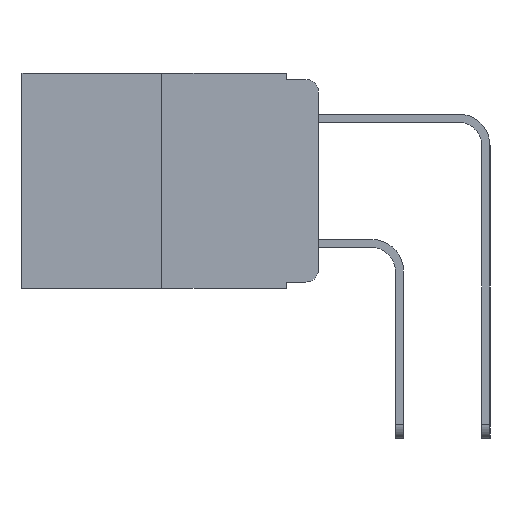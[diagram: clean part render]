
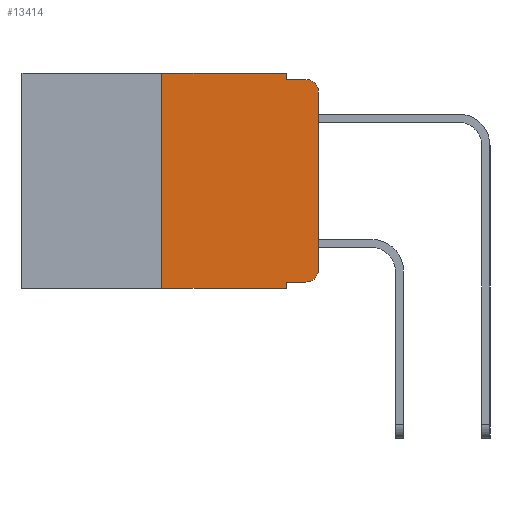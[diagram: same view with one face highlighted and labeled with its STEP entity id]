
A CAD part, left-side view. The second image highlights one B-rep face of the part: STEP entity #13414.
In plain terms, the highlighted planar face has unit normal (-1, 0, 0).
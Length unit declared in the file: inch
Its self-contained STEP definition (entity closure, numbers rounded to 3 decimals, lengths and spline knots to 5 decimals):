
#499 = LINE ( 'NONE', #9097, #16905 ) ;
#1325 = CARTESIAN_POINT ( 'NONE',  ( 0., 0., 0. ) ) ;
#1436 = PLANE ( 'NONE',  #6211 ) ;
#1549 = FACE_OUTER_BOUND ( 'NONE', #18176, .T. ) ;
#1709 = DIRECTION ( 'NONE',  ( 0., 0., -1. ) ) ;
#2256 = VERTEX_POINT ( 'NONE', #17069 ) ;
#2595 = DIRECTION ( 'NONE',  ( 0., 0., -1. ) ) ;
#2981 = CARTESIAN_POINT ( 'NONE',  ( 0., 0.051, -0.01 ) ) ;
#3268 = CARTESIAN_POINT ( 'NONE',  ( 0., 0.02, -0.313 ) ) ;
#3445 = EDGE_CURVE ( 'NONE', #6147, #6642, #19746, .T. ) ;
#4280 = LINE ( 'NONE', #12905, #16364 ) ;
#4606 = VERTEX_POINT ( 'NONE', #10904 ) ;
#4741 = DIRECTION ( 'NONE',  ( 1., 0., 0. ) ) ;
#4770 = ORIENTED_EDGE ( 'NONE', *, *, #20337, .T. ) ;
#4791 = ORIENTED_EDGE ( 'NONE', *, *, #17960, .T. ) ;
#4918 = DIRECTION ( 'NONE',  ( 0., 0., -1. ) ) ;
#5197 = AXIS2_PLACEMENT_3D ( 'NONE', #3268, #14366, #4918 ) ;
#5514 = EDGE_CURVE ( 'NONE', #6147, #6478, #12520, .T. ) ;
#5603 = EDGE_CURVE ( 'NONE', #6843, #2256, #10589, .T. ) ;
#5660 = CARTESIAN_POINT ( 'NONE',  ( 0., 0., -0.03 ) ) ;
#5936 = VERTEX_POINT ( 'NONE', #14163 ) ;
#6147 = VERTEX_POINT ( 'NONE', #11583 ) ;
#6211 = AXIS2_PLACEMENT_3D ( 'NONE', #17232, #4741, #15773 ) ;
#6478 = VERTEX_POINT ( 'NONE', #17294 ) ;
#6642 = VERTEX_POINT ( 'NONE', #16165 ) ;
#6843 = VERTEX_POINT ( 'NONE', #5660 ) ;
#7044 = DIRECTION ( 'NONE',  ( -1., 0., 0. ) ) ;
#7381 = VECTOR ( 'NONE', #11989, 39.37008 ) ;
#7773 = CARTESIAN_POINT ( 'NONE',  ( 0., 0., -0.313 ) ) ;
#8070 = ORIENTED_EDGE ( 'NONE', *, *, #19618, .T. ) ;
#8300 = ORIENTED_EDGE ( 'NONE', *, *, #10717, .F. ) ;
#9097 = CARTESIAN_POINT ( 'NONE',  ( 0., 0.051, -0.333 ) ) ;
#9111 = CARTESIAN_POINT ( 'NONE',  ( 0., 0.051, 0. ) ) ;
#9526 = VERTEX_POINT ( 'NONE', #2981 ) ;
#10340 = CARTESIAN_POINT ( 'NONE',  ( 0., 0.473, -0.343 ) ) ;
#10366 = DIRECTION ( 'NONE',  ( 0., -1., 0. ) ) ;
#10451 = CARTESIAN_POINT ( 'NONE',  ( 0., 0.051, -0.01 ) ) ;
#10589 = CIRCLE ( 'NONE', #18499, 0.02 ) ;
#10717 = EDGE_CURVE ( 'NONE', #4606, #9526, #20004, .T. ) ;
#10824 = VERTEX_POINT ( 'NONE', #7773 ) ;
#10904 = CARTESIAN_POINT ( 'NONE',  ( 0., 0.051, 0. ) ) ;
#11104 = VECTOR ( 'NONE', #10366, 39.37008 ) ;
#11280 = ORIENTED_EDGE ( 'NONE', *, *, #15408, .F. ) ;
#11535 = CARTESIAN_POINT ( 'NONE',  ( 0., 0.25, 0. ) ) ;
#11583 = CARTESIAN_POINT ( 'NONE',  ( 0., 0.25, -0.343 ) ) ;
#11989 = DIRECTION ( 'NONE',  ( 0., -1., 0. ) ) ;
#12031 = VECTOR ( 'NONE', #13077, 39.37008 ) ;
#12056 = LINE ( 'NONE', #10451, #7381 ) ;
#12410 = EDGE_CURVE ( 'NONE', #9526, #2256, #12056, .T. ) ;
#12520 = LINE ( 'NONE', #11535, #12031 ) ;
#12905 = CARTESIAN_POINT ( 'NONE',  ( 0., 0.051, 0. ) ) ;
#13077 = DIRECTION ( 'NONE',  ( 0., 0., 1. ) ) ;
#13414 = ADVANCED_FACE ( 'NONE', ( #1549 ), #1436, .F. ) ;
#13696 = ORIENTED_EDGE ( 'NONE', *, *, #5603, .T. ) ;
#13946 = ORIENTED_EDGE ( 'NONE', *, *, #17488, .F. ) ;
#14104 = DIRECTION ( 'NONE',  ( 0., 0., 1. ) ) ;
#14163 = CARTESIAN_POINT ( 'NONE',  ( 0., 0.02, -0.333 ) ) ;
#14366 = DIRECTION ( 'NONE',  ( -1., 0., 0. ) ) ;
#14423 = ORIENTED_EDGE ( 'NONE', *, *, #5514, .F. ) ;
#15408 = EDGE_CURVE ( 'NONE', #17806, #6642, #4280, .T. ) ;
#15773 = DIRECTION ( 'NONE',  ( 0., 0., -1. ) ) ;
#16165 = CARTESIAN_POINT ( 'NONE',  ( 0., 0.051, -0.343 ) ) ;
#16364 = VECTOR ( 'NONE', #1709, 39.37008 ) ;
#16402 = CARTESIAN_POINT ( 'NONE',  ( 0., 0.02, -0.03 ) ) ;
#16905 = VECTOR ( 'NONE', #18346, 39.37008 ) ;
#17069 = CARTESIAN_POINT ( 'NONE',  ( 0., 0.02, -0.01 ) ) ;
#17232 = CARTESIAN_POINT ( 'NONE',  ( 0., 0.473, 0. ) ) ;
#17294 = CARTESIAN_POINT ( 'NONE',  ( 0., 0.25, 0. ) ) ;
#17462 = CIRCLE ( 'NONE', #5197, 0.02 ) ;
#17488 = EDGE_CURVE ( 'NONE', #6478, #4606, #18435, .T. ) ;
#17799 = CARTESIAN_POINT ( 'NONE',  ( 0., 0.473, 0. ) ) ;
#17806 = VERTEX_POINT ( 'NONE', #19982 ) ;
#17925 = DIRECTION ( 'NONE',  ( 0., 0., -1. ) ) ;
#17960 = EDGE_CURVE ( 'NONE', #5936, #10824, #17462, .T. ) ;
#17963 = VECTOR ( 'NONE', #19323, 39.37008 ) ;
#18176 = EDGE_LOOP ( 'NONE', ( #4770, #13696, #19677, #8300, #13946, #14423, #18491, #11280, #8070, #4791 ) ) ;
#18346 = DIRECTION ( 'NONE',  ( 0., -1., 0. ) ) ;
#18435 = LINE ( 'NONE', #17799, #17963 ) ;
#18491 = ORIENTED_EDGE ( 'NONE', *, *, #3445, .T. ) ;
#18499 = AXIS2_PLACEMENT_3D ( 'NONE', #16402, #7044, #17925 ) ;
#18762 = VECTOR ( 'NONE', #14104, 39.37008 ) ;
#19230 = LINE ( 'NONE', #1325, #18762 ) ;
#19323 = DIRECTION ( 'NONE',  ( 0., -1., 0. ) ) ;
#19532 = VECTOR ( 'NONE', #2595, 39.37008 ) ;
#19618 = EDGE_CURVE ( 'NONE', #17806, #5936, #499, .T. ) ;
#19677 = ORIENTED_EDGE ( 'NONE', *, *, #12410, .F. ) ;
#19746 = LINE ( 'NONE', #10340, #11104 ) ;
#19982 = CARTESIAN_POINT ( 'NONE',  ( 0., 0.051, -0.333 ) ) ;
#20004 = LINE ( 'NONE', #9111, #19532 ) ;
#20337 = EDGE_CURVE ( 'NONE', #10824, #6843, #19230, .T. ) ;
